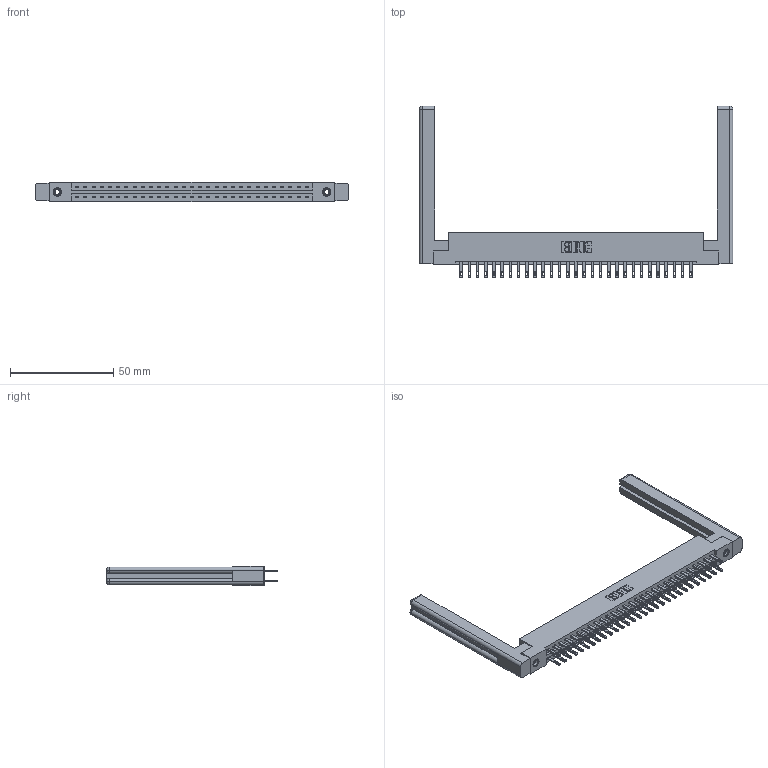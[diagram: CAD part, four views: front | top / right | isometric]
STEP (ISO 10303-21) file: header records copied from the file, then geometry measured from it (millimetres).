
FILE_DESCRIPTION (( 'STEP AP203' ), '1' );
FILE_NAME ('337-058-500-258.STEP', '2019-10-09T19:27:00', ( '' ), ( '' ), 'SwSTEP 2.0', 'SolidWorks 2016', '' );
FILE_SCHEMA (( 'CONFIG_CONTROL_DESIGN' ));
Length unit declared in the file: inch
Products named in the file (5): 345-250-001_345-250-001-102; 337-058-500-258; 345-292-001_345-293-100; 307-220-058; 337 Part_Flush Mounting Lugs - 0.156 Dia-TI
Assembly tree (63 placements, depth 2):
  337-058-500-258
    337 Part_Flush Mounting Lugs - 0.156 Dia-TI
    345-292-001_345-293-100  x58
    345-250-001_345-250-001-102  x2
    307-220-058  x2
Bounding box: 151.54 x 82.94 x 9.4 mm (x, y, z)
Volume: 23116.7 mm3; surface area: 23623 mm2
Topology: 63 solids, 63 shells, 3156 faces, 9539 edges, 6346 vertices
Faces by surface type: plane 2010, cylinder 1122, cone 12, torus 12
Entity records: 26730 total; most frequent: CARTESIAN_POINT 4521, ORIENTED_EDGE 4396, DIRECTION 3886, EDGE_CURVE 2198, VECTOR 2018, LINE 2018, VERTEX_POINT 1458, AXIS2_PLACEMENT_3D 934
